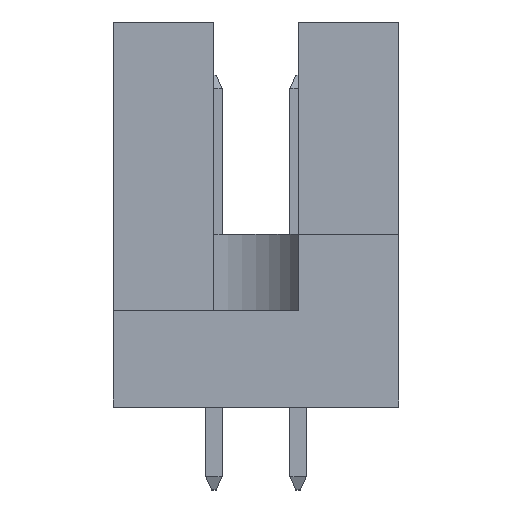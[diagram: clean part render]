
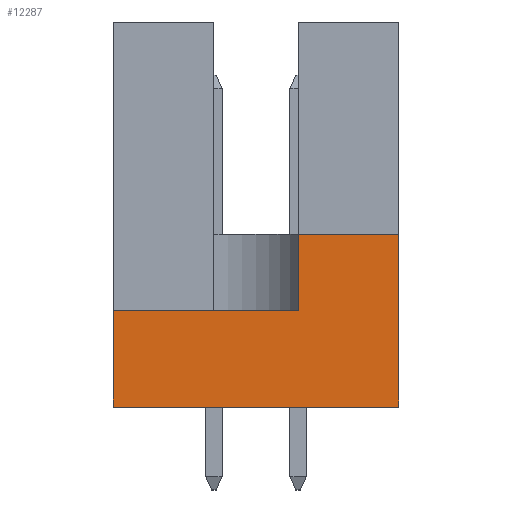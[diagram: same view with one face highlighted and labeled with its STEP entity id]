
A CAD part, left-side view. The second image highlights one B-rep face of the part: STEP entity #12287.
In plain terms, the highlighted planar face has unit normal (-1, 0, 0).
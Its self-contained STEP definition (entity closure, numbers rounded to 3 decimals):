
#58 = DIRECTION ( 'NONE',  ( 0., -1., 0. ) ) ;
#375 = LINE ( 'NONE', #4357, #3067 ) ;
#461 = EDGE_CURVE ( 'NONE', #11370, #3698, #3248, .T. ) ;
#866 = VERTEX_POINT ( 'NONE', #10038 ) ;
#1207 = VECTOR ( 'NONE', #2186, 1000. ) ;
#1257 = CARTESIAN_POINT ( 'NONE',  ( -47.5, -1.27, 19.02 ) ) ;
#1271 = VERTEX_POINT ( 'NONE', #6017 ) ;
#2011 = VECTOR ( 'NONE', #58, 1000. ) ;
#2104 = FACE_OUTER_BOUND ( 'NONE', #11501, .T. ) ;
#2186 = DIRECTION ( 'NONE',  ( 0., 1., 0. ) ) ;
#2595 = EDGE_CURVE ( 'NONE', #3447, #866, #9292, .T. ) ;
#3067 = VECTOR ( 'NONE', #6399, 1000. ) ;
#3248 = LINE ( 'NONE', #7230, #9726 ) ;
#3435 = DIRECTION ( 'NONE',  ( 0., 0., -1. ) ) ;
#3447 = VERTEX_POINT ( 'NONE', #7947 ) ;
#3698 = VERTEX_POINT ( 'NONE', #4611 ) ;
#3718 = ORIENTED_EDGE ( 'NONE', *, *, #461, .T. ) ;
#3965 = ORIENTED_EDGE ( 'NONE', *, *, #5367, .T. ) ;
#4096 = CARTESIAN_POINT ( 'NONE',  ( -47.5, 4.3, 0. ) ) ;
#4115 = VERTEX_POINT ( 'NONE', #5252 ) ;
#4173 = DIRECTION ( 'NONE',  ( 0., 0., -1. ) ) ;
#4239 = ORIENTED_EDGE ( 'NONE', *, *, #2595, .T. ) ;
#4357 = CARTESIAN_POINT ( 'NONE',  ( -47.5, 4.3, 5.2 ) ) ;
#4611 = CARTESIAN_POINT ( 'NONE',  ( -47.5, 4.3, 0. ) ) ;
#4937 = CARTESIAN_POINT ( 'NONE',  ( -47.5, 4.3, 2.9 ) ) ;
#5252 = CARTESIAN_POINT ( 'NONE',  ( -47.5, -4.3, 0. ) ) ;
#5367 = EDGE_CURVE ( 'NONE', #866, #11370, #10747, .T. ) ;
#5576 = ORIENTED_EDGE ( 'NONE', *, *, #11102, .F. ) ;
#5705 = VECTOR ( 'NONE', #8378, 1000. ) ;
#5776 = CARTESIAN_POINT ( 'NONE',  ( -47.5, 4.3, 2.9 ) ) ;
#6017 = CARTESIAN_POINT ( 'NONE',  ( -47.5, -4.3, 5.2 ) ) ;
#6093 = DIRECTION ( 'NONE',  ( 1., 0., 0. ) ) ;
#6399 = DIRECTION ( 'NONE',  ( 0., -1., 0. ) ) ;
#6798 = CARTESIAN_POINT ( 'NONE',  ( -47.5, 4.3, 11.6 ) ) ;
#6933 = PLANE ( 'NONE',  #7218 ) ;
#6987 = LINE ( 'NONE', #9022, #12520 ) ;
#7218 = AXIS2_PLACEMENT_3D ( 'NONE', #6798, #6093, #9809 ) ;
#7230 = CARTESIAN_POINT ( 'NONE',  ( -47.5, 4.3, 11.6 ) ) ;
#7947 = CARTESIAN_POINT ( 'NONE',  ( -47.5, -1.27, 5.2 ) ) ;
#8213 = EDGE_CURVE ( 'NONE', #1271, #4115, #6987, .T. ) ;
#8378 = DIRECTION ( 'NONE',  ( 0., 0., -1. ) ) ;
#9022 = CARTESIAN_POINT ( 'NONE',  ( -47.5, -4.3, 11.6 ) ) ;
#9091 = ORIENTED_EDGE ( 'NONE', *, *, #10251, .T. ) ;
#9292 = LINE ( 'NONE', #1257, #5705 ) ;
#9726 = VECTOR ( 'NONE', #3435, 1000. ) ;
#9809 = DIRECTION ( 'NONE',  ( 0., 0., -1. ) ) ;
#10038 = CARTESIAN_POINT ( 'NONE',  ( -47.5, -1.27, 2.9 ) ) ;
#10111 = LINE ( 'NONE', #4096, #2011 ) ;
#10251 = EDGE_CURVE ( 'NONE', #3698, #4115, #10111, .T. ) ;
#10747 = LINE ( 'NONE', #5776, #1207 ) ;
#11102 = EDGE_CURVE ( 'NONE', #3447, #1271, #375, .T. ) ;
#11370 = VERTEX_POINT ( 'NONE', #4937 ) ;
#11501 = EDGE_LOOP ( 'NONE', ( #5576, #4239, #3965, #3718, #9091, #12035 ) ) ;
#12035 = ORIENTED_EDGE ( 'NONE', *, *, #8213, .F. ) ;
#12287 = ADVANCED_FACE ( 'NONE', ( #2104 ), #6933, .F. ) ;
#12520 = VECTOR ( 'NONE', #4173, 1000. ) ;
